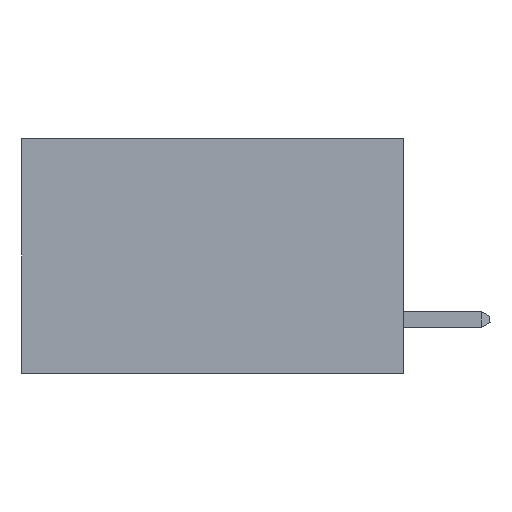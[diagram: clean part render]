
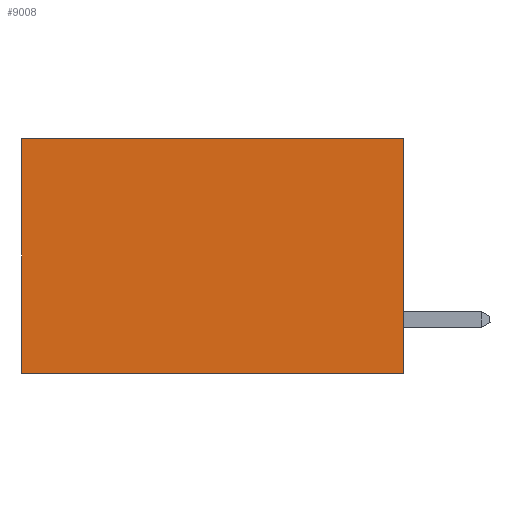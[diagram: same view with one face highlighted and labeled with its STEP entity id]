
A CAD part, left-side view. The second image highlights one B-rep face of the part: STEP entity #9008.
In plain terms, the highlighted planar face has unit normal (-1, 0, 0).
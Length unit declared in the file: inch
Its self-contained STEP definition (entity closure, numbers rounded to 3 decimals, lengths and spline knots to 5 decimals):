
#53 = PLANE ( 'NONE',  #20752 ) ;
#1407 = DIRECTION ( 'NONE',  ( 0., 0., -1. ) ) ;
#2544 = EDGE_CURVE ( 'NONE', #25997, #23173, #24331, .T. ) ;
#4015 = LINE ( 'NONE', #29878, #17310 ) ;
#5896 = ORIENTED_EDGE ( 'NONE', *, *, #2544, .F. ) ;
#6033 = LINE ( 'NONE', #16115, #24666 ) ;
#6527 = FACE_OUTER_BOUND ( 'NONE', #14994, .T. ) ;
#7007 = ORIENTED_EDGE ( 'NONE', *, *, #20000, .T. ) ;
#9008 = ADVANCED_FACE ( 'NONE', ( #6527 ), #53, .F. ) ;
#9777 = VECTOR ( 'NONE', #1407, 39.37008 ) ;
#10251 = CARTESIAN_POINT ( 'NONE',  ( 0.2875, 0.6, 0. ) ) ;
#11949 = DIRECTION ( 'NONE',  ( 1., 0., 0. ) ) ;
#13726 = ORIENTED_EDGE ( 'NONE', *, *, #20497, .F. ) ;
#14138 = EDGE_CURVE ( 'NONE', #21875, #23173, #4015, .T. ) ;
#14994 = EDGE_LOOP ( 'NONE', ( #19316, #5896, #13726, #7007 ) ) ;
#16115 = CARTESIAN_POINT ( 'NONE',  ( 0.2875, 0., 0. ) ) ;
#16188 = DIRECTION ( 'NONE',  ( 0., 0., -1. ) ) ;
#17310 = VECTOR ( 'NONE', #16188, 39.37008 ) ;
#18431 = DIRECTION ( 'NONE',  ( 0., 1., 0. ) ) ;
#19316 = ORIENTED_EDGE ( 'NONE', *, *, #14138, .T. ) ;
#20000 = EDGE_CURVE ( 'NONE', #25091, #21875, #6033, .T. ) ;
#20313 = CARTESIAN_POINT ( 'NONE',  ( 0.2875, 0.6, -0.37 ) ) ;
#20497 = EDGE_CURVE ( 'NONE', #25091, #25997, #28252, .T. ) ;
#20752 = AXIS2_PLACEMENT_3D ( 'NONE', #25822, #11949, #28111 ) ;
#21875 = VERTEX_POINT ( 'NONE', #10251 ) ;
#22118 = DIRECTION ( 'NONE',  ( 0., 1., 0. ) ) ;
#23173 = VERTEX_POINT ( 'NONE', #20313 ) ;
#23984 = CARTESIAN_POINT ( 'NONE',  ( 0.2875, 0., -0.37 ) ) ;
#24331 = LINE ( 'NONE', #26911, #29671 ) ;
#24666 = VECTOR ( 'NONE', #18431, 39.37008 ) ;
#25091 = VERTEX_POINT ( 'NONE', #29599 ) ;
#25822 = CARTESIAN_POINT ( 'NONE',  ( 0.2875, 0., 0. ) ) ;
#25997 = VERTEX_POINT ( 'NONE', #23984 ) ;
#26911 = CARTESIAN_POINT ( 'NONE',  ( 0.2875, 0., -0.37 ) ) ;
#28111 = DIRECTION ( 'NONE',  ( 0., 0., -1. ) ) ;
#28252 = LINE ( 'NONE', #29306, #9777 ) ;
#29306 = CARTESIAN_POINT ( 'NONE',  ( 0.2875, 0., 0. ) ) ;
#29599 = CARTESIAN_POINT ( 'NONE',  ( 0.2875, 0., 0. ) ) ;
#29671 = VECTOR ( 'NONE', #22118, 39.37008 ) ;
#29878 = CARTESIAN_POINT ( 'NONE',  ( 0.2875, 0.6, 0. ) ) ;
